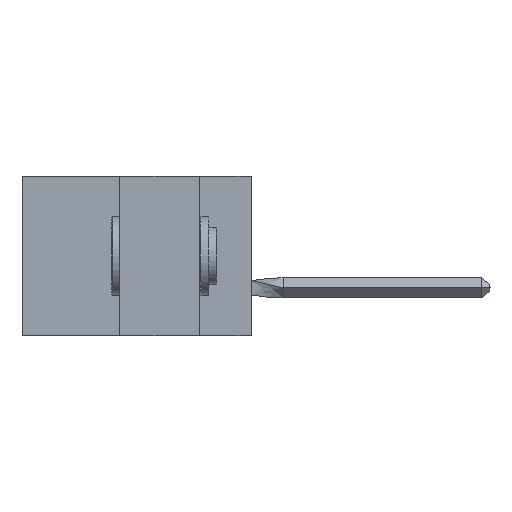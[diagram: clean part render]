
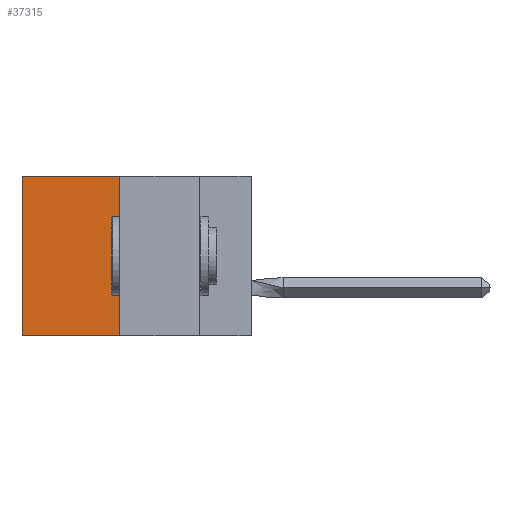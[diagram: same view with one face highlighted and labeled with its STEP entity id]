
A CAD part, left-side view. The second image highlights one B-rep face of the part: STEP entity #37315.
In plain terms, the highlighted planar face has unit normal (-1, 0, 0).
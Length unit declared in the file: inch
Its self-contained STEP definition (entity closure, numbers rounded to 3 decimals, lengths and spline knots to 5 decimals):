
#149 = CARTESIAN_POINT ( 'NONE',  ( 0.305, 0.413, -0.5 ) ) ;
#937 = VECTOR ( 'NONE', #17994, 39.37008 ) ;
#1147 = PLANE ( 'NONE',  #17752 ) ;
#1754 = CARTESIAN_POINT ( 'NONE',  ( 0.305, 0.413, -0.5 ) ) ;
#2436 = VECTOR ( 'NONE', #32342, 39.37008 ) ;
#2632 = VECTOR ( 'NONE', #14324, 39.37008 ) ;
#4315 = DIRECTION ( 'NONE',  ( 0., 0., -1. ) ) ;
#5798 = LINE ( 'NONE', #1754, #26339 ) ;
#7371 = ORIENTED_EDGE ( 'NONE', *, *, #38198, .F. ) ;
#8428 = CARTESIAN_POINT ( 'NONE',  ( 0.305, 0.72, -0.5 ) ) ;
#8576 = EDGE_CURVE ( 'NONE', #30304, #21659, #31536, .T. ) ;
#9486 = LINE ( 'NONE', #8428, #2436 ) ;
#11019 = EDGE_CURVE ( 'NONE', #21659, #34022, #9486, .T. ) ;
#11685 = ORIENTED_EDGE ( 'NONE', *, *, #19577, .F. ) ;
#13764 = ORIENTED_EDGE ( 'NONE', *, *, #8576, .T. ) ;
#14199 = CARTESIAN_POINT ( 'NONE',  ( 0.305, 0.413, 0. ) ) ;
#14324 = DIRECTION ( 'NONE',  ( 0., 1., 0. ) ) ;
#16681 = FACE_OUTER_BOUND ( 'NONE', #28294, .T. ) ;
#16856 = DIRECTION ( 'NONE',  ( 0., 1., 0. ) ) ;
#17752 = AXIS2_PLACEMENT_3D ( 'NONE', #25070, #30991, #4315 ) ;
#17994 = DIRECTION ( 'NONE',  ( 0., 0., -1. ) ) ;
#19577 = EDGE_CURVE ( 'NONE', #30304, #28698, #34964, .T. ) ;
#21659 = VERTEX_POINT ( 'NONE', #30338 ) ;
#22908 = ORIENTED_EDGE ( 'NONE', *, *, #11019, .T. ) ;
#22919 = CARTESIAN_POINT ( 'NONE',  ( 0.305, 0.72, -0.5 ) ) ;
#25070 = CARTESIAN_POINT ( 'NONE',  ( 0.305, 0.413, -0.5 ) ) ;
#26339 = VECTOR ( 'NONE', #16856, 39.37008 ) ;
#28294 = EDGE_LOOP ( 'NONE', ( #22908, #7371, #11685, #13764 ) ) ;
#28698 = VERTEX_POINT ( 'NONE', #29080 ) ;
#29080 = CARTESIAN_POINT ( 'NONE',  ( 0.305, 0.413, -0.5 ) ) ;
#30304 = VERTEX_POINT ( 'NONE', #31342 ) ;
#30338 = CARTESIAN_POINT ( 'NONE',  ( 0.305, 0.72, 0. ) ) ;
#30991 = DIRECTION ( 'NONE',  ( 1., 0., 0. ) ) ;
#31342 = CARTESIAN_POINT ( 'NONE',  ( 0.305, 0.413, 0. ) ) ;
#31536 = LINE ( 'NONE', #14199, #2632 ) ;
#32342 = DIRECTION ( 'NONE',  ( 0., 0., -1. ) ) ;
#34022 = VERTEX_POINT ( 'NONE', #22919 ) ;
#34964 = LINE ( 'NONE', #149, #937 ) ;
#37315 = ADVANCED_FACE ( 'NONE', ( #16681 ), #1147, .F. ) ;
#38198 = EDGE_CURVE ( 'NONE', #28698, #34022, #5798, .T. ) ;
